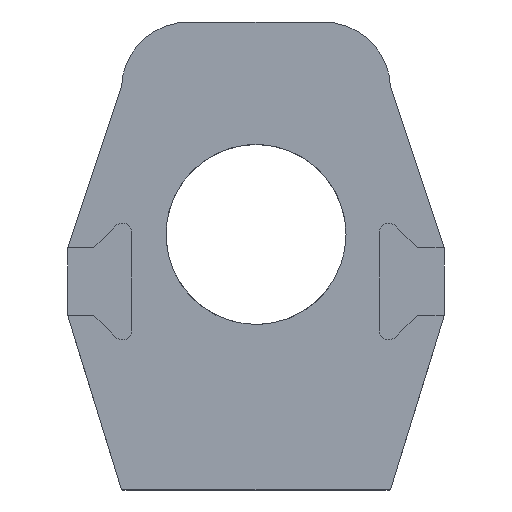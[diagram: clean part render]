
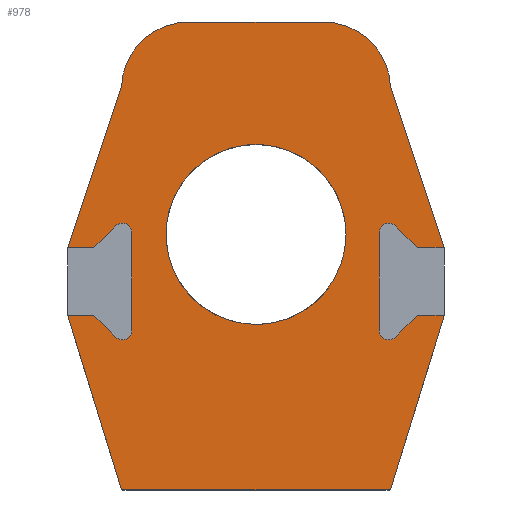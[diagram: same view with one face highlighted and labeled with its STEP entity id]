
A CAD part, front view. The second image highlights one B-rep face of the part: STEP entity #978.
In plain terms, the highlighted planar face has unit normal (0, -1, 0).
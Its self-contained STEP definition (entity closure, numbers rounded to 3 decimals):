
#20=FACE_BOUND('',#154,.T.);
#25=ELLIPSE('',#1047,3.676,2.54);
#27=ELLIPSE('',#1049,3.676,2.54);
#46=CIRCLE('',#1036,0.889);
#48=CIRCLE('',#1040,0.889);
#50=CIRCLE('',#1051,0.889);
#51=CIRCLE('',#1052,0.889);
#52=CIRCLE('',#1053,6.35);
#53=CIRCLE('',#1054,6.35);
#54=CIRCLE('',#1055,8.5);
#55=CIRCLE('',#1056,8.5);
#101=FACE_OUTER_BOUND('',#153,.T.);
#153=EDGE_LOOP('',(#690,#691,#692,#693,#694,#695,#696,#697,#698,#699,#700,
#701,#702,#703,#704,#705,#706,#707,#708,#709,#710,#711,#712,#713));
#154=EDGE_LOOP('',(#714,#715));
#199=LINE('',#1426,#300);
#204=LINE('',#1440,#305);
#208=LINE('',#1452,#309);
#211=LINE('',#1458,#312);
#214=LINE('',#1464,#315);
#223=LINE('',#1502,#324);
#224=LINE('',#1504,#325);
#225=LINE('',#1506,#326);
#226=LINE('',#1510,#327);
#227=LINE('',#1514,#328);
#228=LINE('',#1516,#329);
#229=LINE('',#1518,#330);
#230=LINE('',#1522,#331);
#231=LINE('',#1525,#332);
#232=LINE('',#1526,#333);
#233=LINE('',#1527,#334);
#300=VECTOR('',#1133,10.);
#305=VECTOR('',#1146,10.);
#309=VECTOR('',#1158,10.);
#312=VECTOR('',#1163,10.);
#315=VECTOR('',#1168,10.);
#324=VECTOR('',#1189,10.);
#325=VECTOR('',#1190,10.);
#326=VECTOR('',#1191,10.);
#327=VECTOR('',#1194,10.);
#328=VECTOR('',#1197,10.);
#329=VECTOR('',#1198,10.);
#330=VECTOR('',#1199,10.);
#331=VECTOR('',#1202,10.);
#332=VECTOR('',#1205,10.);
#333=VECTOR('',#1206,10.);
#334=VECTOR('',#1207,10.);
#401=VERTEX_POINT('',#1424);
#402=VERTEX_POINT('',#1425);
#405=VERTEX_POINT('',#1433);
#407=VERTEX_POINT('',#1439);
#409=VERTEX_POINT('',#1445);
#411=VERTEX_POINT('',#1451);
#413=VERTEX_POINT('',#1457);
#415=VERTEX_POINT('',#1463);
#420=VERTEX_POINT('',#1481);
#421=VERTEX_POINT('',#1483);
#424=VERTEX_POINT('',#1495);
#425=VERTEX_POINT('',#1497);
#426=VERTEX_POINT('',#1501);
#427=VERTEX_POINT('',#1503);
#428=VERTEX_POINT('',#1505);
#429=VERTEX_POINT('',#1507);
#430=VERTEX_POINT('',#1509);
#431=VERTEX_POINT('',#1511);
#432=VERTEX_POINT('',#1513);
#433=VERTEX_POINT('',#1515);
#434=VERTEX_POINT('',#1517);
#435=VERTEX_POINT('',#1519);
#436=VERTEX_POINT('',#1521);
#437=VERTEX_POINT('',#1523);
#438=VERTEX_POINT('',#1528);
#439=VERTEX_POINT('',#1529);
#497=EDGE_CURVE('',#401,#402,#199,.T.);
#501=EDGE_CURVE('',#405,#401,#46,.T.);
#504=EDGE_CURVE('',#407,#405,#204,.T.);
#507=EDGE_CURVE('',#409,#407,#48,.T.);
#510=EDGE_CURVE('',#411,#409,#208,.T.);
#513=EDGE_CURVE('',#402,#413,#211,.T.);
#516=EDGE_CURVE('',#415,#411,#214,.T.);
#523=EDGE_CURVE('',#421,#420,#25,.T.);
#527=EDGE_CURVE('',#425,#424,#27,.T.);
#529=EDGE_CURVE('',#424,#426,#223,.T.);
#530=EDGE_CURVE('',#427,#426,#224,.T.);
#531=EDGE_CURVE('',#428,#427,#225,.T.);
#532=EDGE_CURVE('',#429,#428,#50,.T.);
#533=EDGE_CURVE('',#430,#429,#226,.T.);
#534=EDGE_CURVE('',#431,#430,#51,.T.);
#535=EDGE_CURVE('',#432,#431,#227,.T.);
#536=EDGE_CURVE('',#433,#432,#228,.T.);
#537=EDGE_CURVE('',#433,#434,#229,.T.);
#538=EDGE_CURVE('',#434,#435,#52,.T.);
#539=EDGE_CURVE('',#435,#436,#230,.T.);
#540=EDGE_CURVE('',#436,#437,#53,.T.);
#541=EDGE_CURVE('',#437,#415,#231,.T.);
#542=EDGE_CURVE('',#413,#421,#232,.T.);
#543=EDGE_CURVE('',#420,#425,#233,.T.);
#544=EDGE_CURVE('',#438,#439,#54,.T.);
#545=EDGE_CURVE('',#439,#438,#55,.T.);
#690=ORIENTED_EDGE('',*,*,#527,.T.);
#691=ORIENTED_EDGE('',*,*,#529,.T.);
#692=ORIENTED_EDGE('',*,*,#530,.F.);
#693=ORIENTED_EDGE('',*,*,#531,.F.);
#694=ORIENTED_EDGE('',*,*,#532,.F.);
#695=ORIENTED_EDGE('',*,*,#533,.F.);
#696=ORIENTED_EDGE('',*,*,#534,.F.);
#697=ORIENTED_EDGE('',*,*,#535,.F.);
#698=ORIENTED_EDGE('',*,*,#536,.F.);
#699=ORIENTED_EDGE('',*,*,#537,.T.);
#700=ORIENTED_EDGE('',*,*,#538,.T.);
#701=ORIENTED_EDGE('',*,*,#539,.T.);
#702=ORIENTED_EDGE('',*,*,#540,.T.);
#703=ORIENTED_EDGE('',*,*,#541,.T.);
#704=ORIENTED_EDGE('',*,*,#516,.T.);
#705=ORIENTED_EDGE('',*,*,#510,.T.);
#706=ORIENTED_EDGE('',*,*,#507,.T.);
#707=ORIENTED_EDGE('',*,*,#504,.T.);
#708=ORIENTED_EDGE('',*,*,#501,.T.);
#709=ORIENTED_EDGE('',*,*,#497,.T.);
#710=ORIENTED_EDGE('',*,*,#513,.T.);
#711=ORIENTED_EDGE('',*,*,#542,.T.);
#712=ORIENTED_EDGE('',*,*,#523,.T.);
#713=ORIENTED_EDGE('',*,*,#543,.T.);
#714=ORIENTED_EDGE('',*,*,#544,.T.);
#715=ORIENTED_EDGE('',*,*,#545,.T.);
#947=PLANE('',#1050);
#978=ADVANCED_FACE('',(#101,#20),#947,.F.);
#1036=AXIS2_PLACEMENT_3D('',#1434,#1139,#1140);
#1040=AXIS2_PLACEMENT_3D('',#1446,#1151,#1152);
#1047=AXIS2_PLACEMENT_3D('',#1484,#1178,#1179);
#1049=AXIS2_PLACEMENT_3D('',#1498,#1184,#1185);
#1050=AXIS2_PLACEMENT_3D('',#1500,#1187,#1188);
#1051=AXIS2_PLACEMENT_3D('',#1508,#1192,#1193);
#1052=AXIS2_PLACEMENT_3D('',#1512,#1195,#1196);
#1053=AXIS2_PLACEMENT_3D('',#1520,#1200,#1201);
#1054=AXIS2_PLACEMENT_3D('',#1524,#1203,#1204);
#1055=AXIS2_PLACEMENT_3D('',#1530,#1208,#1209);
#1056=AXIS2_PLACEMENT_3D('',#1531,#1210,#1211);
#1133=DIRECTION('',(-0.707,0.,0.707));
#1139=DIRECTION('center_axis',(0.,1.,0.));
#1140=DIRECTION('ref_axis',(1.,0.,0.));
#1146=DIRECTION('',(0.,0.,-1.));
#1151=DIRECTION('center_axis',(0.,1.,0.));
#1152=DIRECTION('ref_axis',(-0.707,0.,0.707));
#1158=DIRECTION('',(0.707,0.,0.707));
#1163=DIRECTION('',(-1.,0.,0.));
#1168=DIRECTION('',(1.,0.,0.001));
#1178=DIRECTION('center_axis',(0.,-1.,0.));
#1179=DIRECTION('ref_axis',(0.294,0.,-0.956));
#1184=DIRECTION('center_axis',(0.,-1.,0.));
#1185=DIRECTION('ref_axis',(-0.294,0.,-0.956));
#1187=DIRECTION('center_axis',(0.,1.,0.));
#1188=DIRECTION('ref_axis',(-1.,0.,0.));
#1189=DIRECTION('',(0.294,0.,0.956));
#1190=DIRECTION('',(1.,0.,0.));
#1191=DIRECTION('',(0.707,0.,0.707));
#1192=DIRECTION('center_axis',(0.,-1.,0.));
#1193=DIRECTION('ref_axis',(0.707,0.,-0.707));
#1194=DIRECTION('',(0.,0.,-1.));
#1195=DIRECTION('center_axis',(0.,-1.,0.));
#1196=DIRECTION('ref_axis',(-1.,0.,0.));
#1197=DIRECTION('',(-0.707,0.,0.707));
#1198=DIRECTION('',(-1.,0.,0.001));
#1199=DIRECTION('',(-0.316,0.,0.949));
#1200=DIRECTION('center_axis',(0.,-1.,0.));
#1201=DIRECTION('ref_axis',(0.999,0.,0.04));
#1202=DIRECTION('',(-1.,0.,0.));
#1203=DIRECTION('center_axis',(0.,-1.,0.));
#1204=DIRECTION('ref_axis',(-0.999,0.,0.04));
#1205=DIRECTION('',(-0.316,0.,-0.949));
#1206=DIRECTION('',(0.294,0.,-0.956));
#1207=DIRECTION('',(1.,0.,0.));
#1208=DIRECTION('center_axis',(0.,1.,0.));
#1209=DIRECTION('ref_axis',(-1.,0.,0.));
#1210=DIRECTION('center_axis',(0.,1.,0.));
#1211=DIRECTION('ref_axis',(-1.,0.,0.));
#1424=CARTESIAN_POINT('',(-13.243,124.66,1.736));
#1425=CARTESIAN_POINT('',(-15.317,124.66,3.81));
#1426=CARTESIAN_POINT('',(-11.086,124.66,-0.422));
#1433=CARTESIAN_POINT('',(-11.725,124.66,2.364));
#1434=CARTESIAN_POINT('Origin',(-12.614,124.66,2.364));
#1439=CARTESIAN_POINT('',(-11.725,124.66,11.609));
#1440=CARTESIAN_POINT('',(-11.725,124.66,8.979));
#1445=CARTESIAN_POINT('',(-13.243,124.66,12.238));
#1446=CARTESIAN_POINT('Origin',(-12.614,124.66,11.609));
#1451=CARTESIAN_POINT('',(-15.317,124.66,10.163));
#1452=CARTESIAN_POINT('',(-12.441,124.66,13.039));
#1457=CARTESIAN_POINT('',(-17.78,124.66,3.81));
#1458=CARTESIAN_POINT('',(-7.659,124.66,3.81));
#1463=CARTESIAN_POINT('',(-17.78,124.66,10.16));
#1464=CARTESIAN_POINT('',(-8.892,124.66,10.171));
#1481=CARTESIAN_POINT('',(-12.69,124.66,-12.699));
#1483=CARTESIAN_POINT('',(-12.794,124.66,-12.394));
#1484=CARTESIAN_POINT('Origin',(-10.366,124.66,-11.647));
#1495=CARTESIAN_POINT('',(12.794,124.66,-12.394));
#1497=CARTESIAN_POINT('',(12.69,124.66,-12.699));
#1498=CARTESIAN_POINT('Origin',(10.366,124.66,-11.647));
#1500=CARTESIAN_POINT('Origin',(0.,124.66,6.35));
#1501=CARTESIAN_POINT('',(17.78,124.66,3.81));
#1502=CARTESIAN_POINT('',(17.368,124.66,2.471));
#1503=CARTESIAN_POINT('',(15.24,124.66,3.81));
#1504=CARTESIAN_POINT('',(8.89,124.66,3.81));
#1505=CARTESIAN_POINT('',(13.166,124.66,1.736));
#1506=CARTESIAN_POINT('',(12.065,124.66,0.635));
#1507=CARTESIAN_POINT('',(11.648,124.66,2.364));
#1508=CARTESIAN_POINT('Origin',(12.537,124.66,2.364));
#1509=CARTESIAN_POINT('',(11.648,124.66,11.609));
#1510=CARTESIAN_POINT('',(11.648,124.66,4.357));
#1511=CARTESIAN_POINT('',(13.166,124.66,12.238));
#1512=CARTESIAN_POINT('Origin',(12.537,124.66,11.609));
#1513=CARTESIAN_POINT('',(15.24,124.66,10.163));
#1514=CARTESIAN_POINT('',(11.346,124.66,14.057));
#1515=CARTESIAN_POINT('',(17.78,124.66,10.16));
#1516=CARTESIAN_POINT('',(7.622,124.66,10.172));
#1517=CARTESIAN_POINT('',(12.7,124.66,25.4));
#1518=CARTESIAN_POINT('',(14.923,124.66,18.733));
#1519=CARTESIAN_POINT('',(6.355,124.66,31.496));
#1520=CARTESIAN_POINT('Origin',(6.355,124.66,25.146));
#1521=CARTESIAN_POINT('',(-6.355,124.66,31.496));
#1522=CARTESIAN_POINT('',(-6.35,124.66,31.496));
#1523=CARTESIAN_POINT('',(-12.7,124.66,25.4));
#1524=CARTESIAN_POINT('Origin',(-6.355,124.66,25.146));
#1525=CARTESIAN_POINT('',(-17.463,124.66,11.113));
#1526=CARTESIAN_POINT('',(-14.828,124.66,-5.784));
#1527=CARTESIAN_POINT('',(6.35,124.66,-12.699));
#1528=CARTESIAN_POINT('',(8.064,124.66,14.118));
#1529=CARTESIAN_POINT('',(8.5,124.66,11.43));
#1530=CARTESIAN_POINT('Origin',(0.,124.66,11.43));
#1531=CARTESIAN_POINT('Origin',(0.,124.66,11.43));
